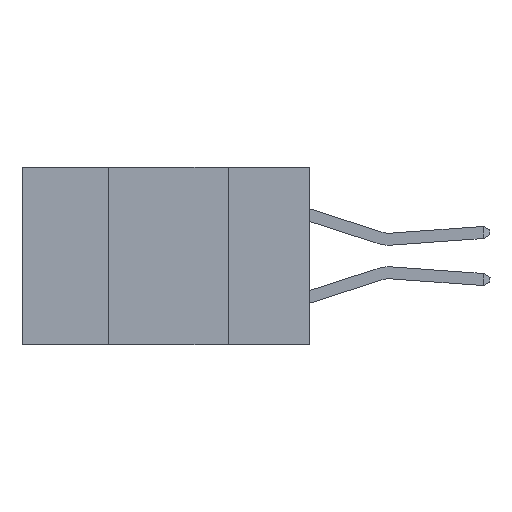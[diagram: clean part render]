
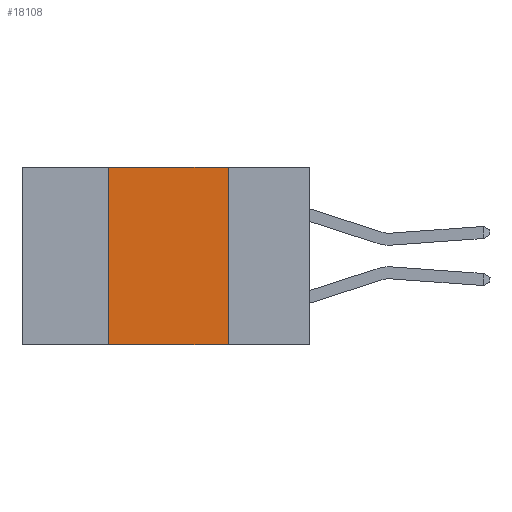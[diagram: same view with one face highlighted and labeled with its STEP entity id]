
A CAD part, left-side view. The second image highlights one B-rep face of the part: STEP entity #18108.
In plain terms, the highlighted planar face has unit normal (-1, 0, 0).
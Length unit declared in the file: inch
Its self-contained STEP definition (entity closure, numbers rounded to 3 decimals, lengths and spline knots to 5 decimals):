
#6 = CARTESIAN_POINT ( 'NONE',  ( 0., 0.42, 0. ) ) ;
#102 = CARTESIAN_POINT ( 'NONE',  ( 0., 0.17, -0.37 ) ) ;
#220 = ORIENTED_EDGE ( 'NONE', *, *, #6633, .F. ) ;
#469 = EDGE_LOOP ( 'NONE', ( #220, #790, #2477, #17657 ) ) ;
#790 = ORIENTED_EDGE ( 'NONE', *, *, #19743, .F. ) ;
#869 = VECTOR ( 'NONE', #11860, 39.37008 ) ;
#1568 = FACE_OUTER_BOUND ( 'NONE', #469, .T. ) ;
#1991 = PLANE ( 'NONE',  #15764 ) ;
#2477 = ORIENTED_EDGE ( 'NONE', *, *, #19173, .F. ) ;
#3792 = VERTEX_POINT ( 'NONE', #14381 ) ;
#3797 = DIRECTION ( 'NONE',  ( 0., 0., -1. ) ) ;
#5673 = LINE ( 'NONE', #11886, #869 ) ;
#6511 = CARTESIAN_POINT ( 'NONE',  ( 0., 0.6, 0. ) ) ;
#6633 = EDGE_CURVE ( 'NONE', #3792, #14320, #5673, .T. ) ;
#7150 = LINE ( 'NONE', #18965, #7714 ) ;
#7714 = VECTOR ( 'NONE', #22496, 39.37008 ) ;
#8304 = CARTESIAN_POINT ( 'NONE',  ( 0., 0.6, -0.37 ) ) ;
#9069 = VECTOR ( 'NONE', #10124, 39.37008 ) ;
#10124 = DIRECTION ( 'NONE',  ( 0., -1., 0. ) ) ;
#11675 = VERTEX_POINT ( 'NONE', #6 ) ;
#11765 = VERTEX_POINT ( 'NONE', #14627 ) ;
#11860 = DIRECTION ( 'NONE',  ( 0., 0., -1. ) ) ;
#11886 = CARTESIAN_POINT ( 'NONE',  ( 0., 0.17, -0.37 ) ) ;
#12775 = CARTESIAN_POINT ( 'NONE',  ( 0., 0.6, 0. ) ) ;
#14320 = VERTEX_POINT ( 'NONE', #102 ) ;
#14381 = CARTESIAN_POINT ( 'NONE',  ( 0., 0.17, 0. ) ) ;
#14420 = LINE ( 'NONE', #6511, #9069 ) ;
#14560 = DIRECTION ( 'NONE',  ( 1., 0., 0. ) ) ;
#14627 = CARTESIAN_POINT ( 'NONE',  ( 0., 0.42, -0.37 ) ) ;
#15764 = AXIS2_PLACEMENT_3D ( 'NONE', #12775, #14560, #3797 ) ;
#17229 = DIRECTION ( 'NONE',  ( 0., -1., 0. ) ) ;
#17454 = LINE ( 'NONE', #8304, #22172 ) ;
#17657 = ORIENTED_EDGE ( 'NONE', *, *, #20195, .T. ) ;
#18108 = ADVANCED_FACE ( 'NONE', ( #1568 ), #1991, .F. ) ;
#18965 = CARTESIAN_POINT ( 'NONE',  ( 0., 0.42, -0.37 ) ) ;
#19173 = EDGE_CURVE ( 'NONE', #11765, #11675, #7150, .T. ) ;
#19743 = EDGE_CURVE ( 'NONE', #11675, #3792, #14420, .T. ) ;
#20195 = EDGE_CURVE ( 'NONE', #11765, #14320, #17454, .T. ) ;
#22172 = VECTOR ( 'NONE', #17229, 39.37008 ) ;
#22496 = DIRECTION ( 'NONE',  ( 0., 0., 1. ) ) ;
